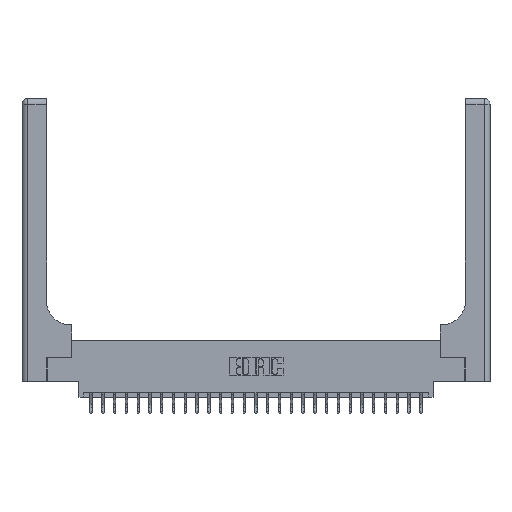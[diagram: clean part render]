
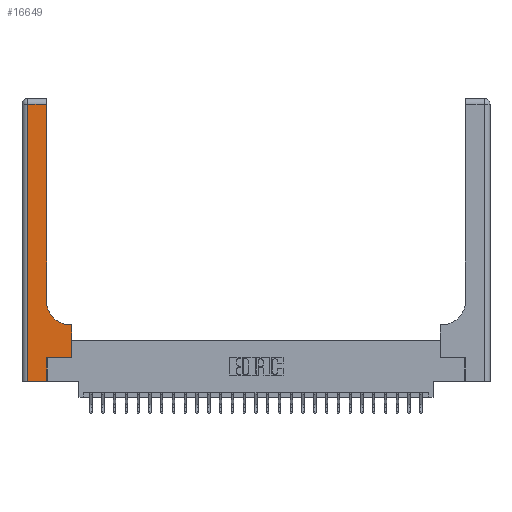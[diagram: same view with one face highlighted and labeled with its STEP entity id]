
A CAD part, top view. The second image highlights one B-rep face of the part: STEP entity #16649.
In plain terms, the highlighted planar face has unit normal (0, 0, 1).
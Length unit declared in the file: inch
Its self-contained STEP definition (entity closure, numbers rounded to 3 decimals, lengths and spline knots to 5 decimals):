
#419 = LINE ( 'NONE', #17592, #16591 ) ;
#440 = EDGE_LOOP ( 'NONE', ( #17062, #25028, #8740, #21028, #9698, #22214, #1439, #6043, #8575 ) ) ;
#443 = EDGE_CURVE ( 'NONE', #16915, #20491, #17586, .T. ) ;
#1439 = ORIENTED_EDGE ( 'NONE', *, *, #15884, .T. ) ;
#1818 = CARTESIAN_POINT ( 'NONE',  ( 0.51, 0.85, 0.37 ) ) ;
#1914 = CARTESIAN_POINT ( 'NONE',  ( 0.265, 0.25, 0.37 ) ) ;
#2613 = CARTESIAN_POINT ( 'NONE',  ( 0.265, 0.25, 0.37 ) ) ;
#2651 = EDGE_CURVE ( 'NONE', #9146, #3704, #11736, .T. ) ;
#2833 = LINE ( 'NONE', #26198, #23772 ) ;
#3458 = CARTESIAN_POINT ( 'NONE',  ( 0.26, 2.94, 0.37 ) ) ;
#3584 = CARTESIAN_POINT ( 'NONE',  ( 0.06, 0., 0.37 ) ) ;
#3704 = VERTEX_POINT ( 'NONE', #24788 ) ;
#3817 = DIRECTION ( 'NONE',  ( 1., 0., 0. ) ) ;
#4155 = FACE_OUTER_BOUND ( 'NONE', #440, .T. ) ;
#4431 = CARTESIAN_POINT ( 'NONE',  ( 0.528, 0.6, 0.37 ) ) ;
#4631 = DIRECTION ( 'NONE',  ( 1., 0., 0. ) ) ;
#5303 = CARTESIAN_POINT ( 'NONE',  ( 0.26, 0.6, 0.37 ) ) ;
#6043 = ORIENTED_EDGE ( 'NONE', *, *, #9062, .T. ) ;
#6357 = VECTOR ( 'NONE', #8919, 39.37008 ) ;
#6865 = CARTESIAN_POINT ( 'NONE',  ( 0.26, 0.85, 0.37 ) ) ;
#7393 = LINE ( 'NONE', #23800, #22979 ) ;
#8575 = ORIENTED_EDGE ( 'NONE', *, *, #443, .T. ) ;
#8740 = ORIENTED_EDGE ( 'NONE', *, *, #22552, .T. ) ;
#8919 = DIRECTION ( 'NONE',  ( -1., 0., 0. ) ) ;
#9062 = EDGE_CURVE ( 'NONE', #22827, #16915, #11942, .T. ) ;
#9146 = VERTEX_POINT ( 'NONE', #3458 ) ;
#9499 = CARTESIAN_POINT ( 'NONE',  ( 0.06, 3., 0.37 ) ) ;
#9673 = DIRECTION ( 'NONE',  ( 1., 0., 0. ) ) ;
#9698 = ORIENTED_EDGE ( 'NONE', *, *, #11284, .T. ) ;
#10184 = DIRECTION ( 'NONE',  ( -1., 0., 0. ) ) ;
#10662 = CARTESIAN_POINT ( 'NONE',  ( 0.528, 0.25, 0.37 ) ) ;
#10678 = AXIS2_PLACEMENT_3D ( 'NONE', #20240, #22365, #10184 ) ;
#11284 = EDGE_CURVE ( 'NONE', #15916, #13395, #17566, .T. ) ;
#11736 = LINE ( 'NONE', #19095, #6357 ) ;
#11942 = LINE ( 'NONE', #5303, #23399 ) ;
#12157 = VECTOR ( 'NONE', #18241, 39.37008 ) ;
#13372 = AXIS2_PLACEMENT_3D ( 'NONE', #1818, #15973, #3817 ) ;
#13395 = VERTEX_POINT ( 'NONE', #1914 ) ;
#13571 = DIRECTION ( 'NONE',  ( 0., -1., 0. ) ) ;
#13857 = VECTOR ( 'NONE', #13571, 39.37008 ) ;
#14490 = LINE ( 'NONE', #9499, #13857 ) ;
#14892 = LINE ( 'NONE', #2613, #25078 ) ;
#14996 = EDGE_CURVE ( 'NONE', #20740, #15916, #7393, .T. ) ;
#15121 = CARTESIAN_POINT ( 'NONE',  ( 0.51, 0.6, 0.37 ) ) ;
#15884 = EDGE_CURVE ( 'NONE', #22271, #22827, #419, .T. ) ;
#15916 = VERTEX_POINT ( 'NONE', #19736 ) ;
#15973 = DIRECTION ( 'NONE',  ( 0., 0., -1. ) ) ;
#16089 = DIRECTION ( 'NONE',  ( 0., 1., 0. ) ) ;
#16169 = CARTESIAN_POINT ( 'NONE',  ( 0.265, 0., 0.37 ) ) ;
#16591 = VECTOR ( 'NONE', #21696, 39.37008 ) ;
#16649 = ADVANCED_FACE ( 'NONE', ( #4155 ), #20337, .F. ) ;
#16915 = VERTEX_POINT ( 'NONE', #15121 ) ;
#17062 = ORIENTED_EDGE ( 'NONE', *, *, #20837, .T. ) ;
#17566 = LINE ( 'NONE', #16169, #12157 ) ;
#17586 = CIRCLE ( 'NONE', #13372, 0.25 ) ;
#17592 = CARTESIAN_POINT ( 'NONE',  ( 0.528, 0.25, 0.37 ) ) ;
#18241 = DIRECTION ( 'NONE',  ( 0., 1., 0. ) ) ;
#19095 = CARTESIAN_POINT ( 'NONE',  ( 0., 2.94, 0.37 ) ) ;
#19538 = DIRECTION ( 'NONE',  ( -1., 0., 0. ) ) ;
#19736 = CARTESIAN_POINT ( 'NONE',  ( 0.265, 0., 0.37 ) ) ;
#20240 = CARTESIAN_POINT ( 'NONE',  ( 0., 3., 0.37 ) ) ;
#20337 = PLANE ( 'NONE',  #10678 ) ;
#20491 = VERTEX_POINT ( 'NONE', #6865 ) ;
#20740 = VERTEX_POINT ( 'NONE', #3584 ) ;
#20837 = EDGE_CURVE ( 'NONE', #20491, #9146, #2833, .T. ) ;
#21010 = EDGE_CURVE ( 'NONE', #13395, #22271, #14892, .T. ) ;
#21028 = ORIENTED_EDGE ( 'NONE', *, *, #14996, .T. ) ;
#21696 = DIRECTION ( 'NONE',  ( 0., 1., 0. ) ) ;
#22214 = ORIENTED_EDGE ( 'NONE', *, *, #21010, .T. ) ;
#22271 = VERTEX_POINT ( 'NONE', #10662 ) ;
#22365 = DIRECTION ( 'NONE',  ( 0., 0., -1. ) ) ;
#22552 = EDGE_CURVE ( 'NONE', #3704, #20740, #14490, .T. ) ;
#22827 = VERTEX_POINT ( 'NONE', #4431 ) ;
#22979 = VECTOR ( 'NONE', #9673, 39.37008 ) ;
#23399 = VECTOR ( 'NONE', #19538, 39.37008 ) ;
#23772 = VECTOR ( 'NONE', #16089, 39.37008 ) ;
#23800 = CARTESIAN_POINT ( 'NONE',  ( 0., 0., 0.37 ) ) ;
#24788 = CARTESIAN_POINT ( 'NONE',  ( 0.06, 2.94, 0.37 ) ) ;
#25028 = ORIENTED_EDGE ( 'NONE', *, *, #2651, .T. ) ;
#25078 = VECTOR ( 'NONE', #4631, 39.37008 ) ;
#26198 = CARTESIAN_POINT ( 'NONE',  ( 0.26, 3., 0.37 ) ) ;
